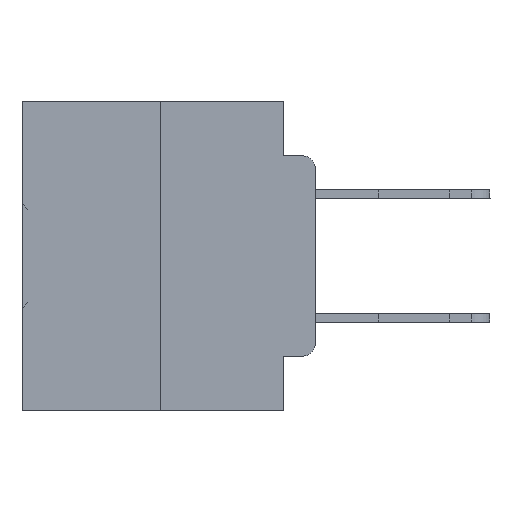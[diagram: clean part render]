
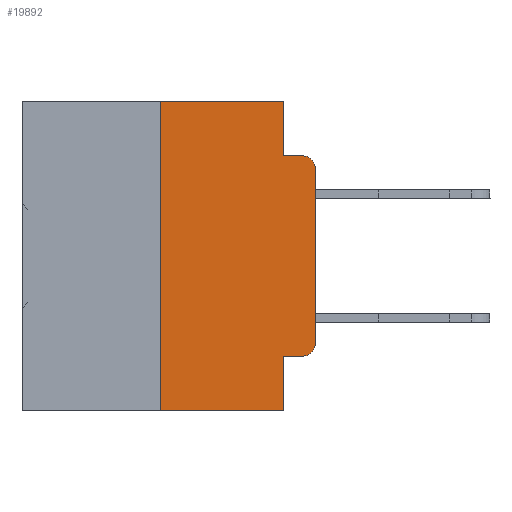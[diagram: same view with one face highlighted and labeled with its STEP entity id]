
A CAD part, left-side view. The second image highlights one B-rep face of the part: STEP entity #19892.
In plain terms, the highlighted planar face has unit normal (-1, 0, 0).
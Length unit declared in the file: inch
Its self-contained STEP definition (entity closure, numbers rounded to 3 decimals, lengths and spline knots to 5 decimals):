
#46 = ORIENTED_EDGE ( 'NONE', *, *, #6232, .T. ) ;
#57 = EDGE_LOOP ( 'NONE', ( #30653, #27686, #6244, #18589, #6374, #28296, #46, #13170, #18803, #18800 ) ) ;
#352 = LINE ( 'NONE', #11789, #1329 ) ;
#791 = VECTOR ( 'NONE', #20193, 39.37008 ) ;
#838 = AXIS2_PLACEMENT_3D ( 'NONE', #21607, #18815, #27427 ) ;
#1329 = VECTOR ( 'NONE', #31998, 39.37008 ) ;
#1484 = VECTOR ( 'NONE', #34296, 39.37008 ) ;
#2039 = CARTESIAN_POINT ( 'NONE',  ( 0., 0.051, -0.0885 ) ) ;
#2096 = CARTESIAN_POINT ( 'NONE',  ( 0., 0.051, -0.0885 ) ) ;
#2108 = EDGE_CURVE ( 'NONE', #14115, #4244, #26207, .T. ) ;
#2551 = EDGE_CURVE ( 'NONE', #31437, #25764, #352, .T. ) ;
#2588 = LINE ( 'NONE', #2039, #5445 ) ;
#3170 = VECTOR ( 'NONE', #18204, 39.37008 ) ;
#3551 = CARTESIAN_POINT ( 'NONE',  ( 0., 0.02, -0.1085 ) ) ;
#3558 = LINE ( 'NONE', #14964, #791 ) ;
#3935 = AXIS2_PLACEMENT_3D ( 'NONE', #19383, #8177, #36263 ) ;
#4244 = VERTEX_POINT ( 'NONE', #12395 ) ;
#5344 = CARTESIAN_POINT ( 'NONE',  ( 0., 0., -0.3915 ) ) ;
#5445 = VECTOR ( 'NONE', #25393, 39.37008 ) ;
#5499 = VECTOR ( 'NONE', #23326, 39.37008 ) ;
#6108 = EDGE_CURVE ( 'NONE', #30948, #25462, #2588, .T. ) ;
#6232 = EDGE_CURVE ( 'NONE', #14115, #25764, #9133, .T. ) ;
#6244 = ORIENTED_EDGE ( 'NONE', *, *, #6108, .F. ) ;
#6374 = ORIENTED_EDGE ( 'NONE', *, *, #33887, .F. ) ;
#6999 = DIRECTION ( 'NONE',  ( 0., -1., 0. ) ) ;
#8177 = DIRECTION ( 'NONE',  ( 1., 0., 0. ) ) ;
#8361 = PLANE ( 'NONE',  #3935 ) ;
#8878 = CIRCLE ( 'NONE', #32790, 0.02 ) ;
#9023 = DIRECTION ( 'NONE',  ( 0., 0., 1. ) ) ;
#9133 = LINE ( 'NONE', #14364, #5499 ) ;
#9230 = VERTEX_POINT ( 'NONE', #21856 ) ;
#11238 = DIRECTION ( 'NONE',  ( 0., 0., -1. ) ) ;
#11406 = CARTESIAN_POINT ( 'NONE',  ( 0., 0.02, -0.4115 ) ) ;
#11789 = CARTESIAN_POINT ( 'NONE',  ( 0., 0.051, 0. ) ) ;
#12395 = CARTESIAN_POINT ( 'NONE',  ( 0., 0.25, 0. ) ) ;
#12757 = CARTESIAN_POINT ( 'NONE',  ( 0., 0.051, -0.5 ) ) ;
#13170 = ORIENTED_EDGE ( 'NONE', *, *, #2551, .F. ) ;
#14015 = VERTEX_POINT ( 'NONE', #11406 ) ;
#14115 = VERTEX_POINT ( 'NONE', #35160 ) ;
#14216 = DIRECTION ( 'NONE',  ( -1., 0., 0. ) ) ;
#14364 = CARTESIAN_POINT ( 'NONE',  ( 0., 0.473, -0.5 ) ) ;
#14850 = VERTEX_POINT ( 'NONE', #32866 ) ;
#14964 = CARTESIAN_POINT ( 'NONE',  ( 0., 0., 0. ) ) ;
#17830 = EDGE_CURVE ( 'NONE', #36623, #14850, #3558, .T. ) ;
#18204 = DIRECTION ( 'NONE',  ( 0., 0., -1. ) ) ;
#18589 = ORIENTED_EDGE ( 'NONE', *, *, #32193, .F. ) ;
#18800 = ORIENTED_EDGE ( 'NONE', *, *, #33430, .T. ) ;
#18803 = ORIENTED_EDGE ( 'NONE', *, *, #22203, .T. ) ;
#18815 = DIRECTION ( 'NONE',  ( -1., 0., 0. ) ) ;
#18934 = VECTOR ( 'NONE', #6999, 39.37008 ) ;
#19188 = CARTESIAN_POINT ( 'NONE',  ( 0., 0.02, -0.0885 ) ) ;
#19383 = CARTESIAN_POINT ( 'NONE',  ( 0., 0.473, 0. ) ) ;
#19892 = ADVANCED_FACE ( 'NONE', ( #33261 ), #8361, .F. ) ;
#20193 = DIRECTION ( 'NONE',  ( 0., 0., 1. ) ) ;
#20581 = CARTESIAN_POINT ( 'NONE',  ( 0., 0.25, 0. ) ) ;
#21607 = CARTESIAN_POINT ( 'NONE',  ( 0., 0.02, -0.3915 ) ) ;
#21856 = CARTESIAN_POINT ( 'NONE',  ( 0., 0.051, 0. ) ) ;
#22203 = EDGE_CURVE ( 'NONE', #31437, #14015, #30195, .T. ) ;
#22293 = CARTESIAN_POINT ( 'NONE',  ( 0., 0.473, 0. ) ) ;
#23326 = DIRECTION ( 'NONE',  ( 0., -1., 0. ) ) ;
#24352 = EDGE_CURVE ( 'NONE', #14850, #25462, #8878, .T. ) ;
#24828 = CARTESIAN_POINT ( 'NONE',  ( 0., 0.051, -0.4115 ) ) ;
#25393 = DIRECTION ( 'NONE',  ( 0., -1., 0. ) ) ;
#25462 = VERTEX_POINT ( 'NONE', #19188 ) ;
#25764 = VERTEX_POINT ( 'NONE', #12757 ) ;
#26207 = LINE ( 'NONE', #20581, #32187 ) ;
#26630 = CARTESIAN_POINT ( 'NONE',  ( 0., 0.051, -0.4115 ) ) ;
#27427 = DIRECTION ( 'NONE',  ( 0., 0., -1. ) ) ;
#27686 = ORIENTED_EDGE ( 'NONE', *, *, #24352, .T. ) ;
#28296 = ORIENTED_EDGE ( 'NONE', *, *, #2108, .F. ) ;
#29633 = LINE ( 'NONE', #32080, #3170 ) ;
#30195 = LINE ( 'NONE', #26630, #18934 ) ;
#30653 = ORIENTED_EDGE ( 'NONE', *, *, #17830, .T. ) ;
#30948 = VERTEX_POINT ( 'NONE', #2096 ) ;
#31125 = LINE ( 'NONE', #22293, #1484 ) ;
#31342 = CIRCLE ( 'NONE', #838, 0.02 ) ;
#31437 = VERTEX_POINT ( 'NONE', #24828 ) ;
#31998 = DIRECTION ( 'NONE',  ( 0., 0., -1. ) ) ;
#32080 = CARTESIAN_POINT ( 'NONE',  ( 0., 0.051, 0. ) ) ;
#32187 = VECTOR ( 'NONE', #9023, 39.37008 ) ;
#32193 = EDGE_CURVE ( 'NONE', #9230, #30948, #29633, .T. ) ;
#32790 = AXIS2_PLACEMENT_3D ( 'NONE', #3551, #14216, #11238 ) ;
#32866 = CARTESIAN_POINT ( 'NONE',  ( 0., 0., -0.1085 ) ) ;
#33261 = FACE_OUTER_BOUND ( 'NONE', #57, .T. ) ;
#33430 = EDGE_CURVE ( 'NONE', #14015, #36623, #31342, .T. ) ;
#33887 = EDGE_CURVE ( 'NONE', #4244, #9230, #31125, .T. ) ;
#34296 = DIRECTION ( 'NONE',  ( 0., -1., 0. ) ) ;
#35160 = CARTESIAN_POINT ( 'NONE',  ( 0., 0.25, -0.5 ) ) ;
#36263 = DIRECTION ( 'NONE',  ( 0., 0., -1. ) ) ;
#36623 = VERTEX_POINT ( 'NONE', #5344 ) ;
